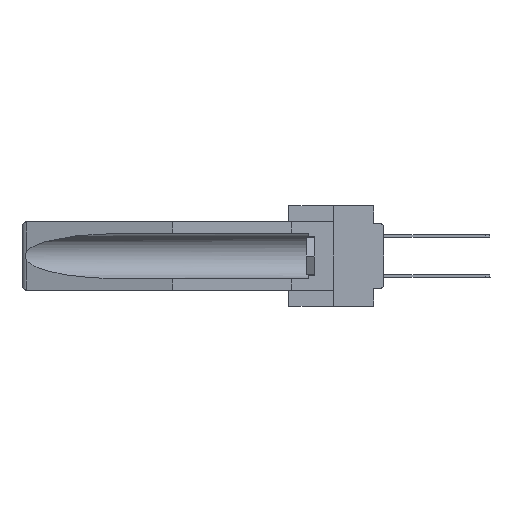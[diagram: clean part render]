
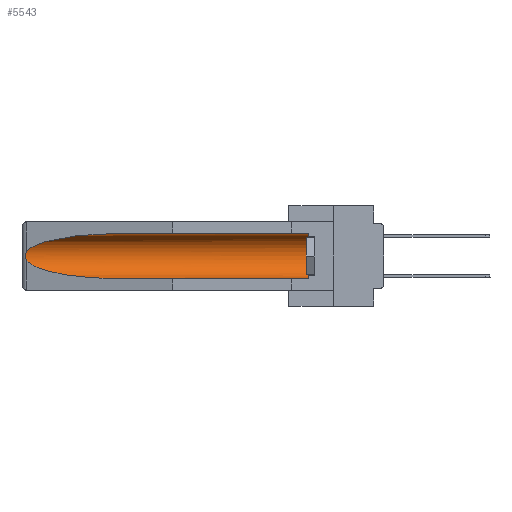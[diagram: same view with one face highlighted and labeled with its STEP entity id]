
A CAD part, left-side view. The second image highlights one B-rep face of the part: STEP entity #5543.
In plain terms, the highlighted cylindrical face has radius 2.857 mm (diameter 5.715 mm), a partial arc.
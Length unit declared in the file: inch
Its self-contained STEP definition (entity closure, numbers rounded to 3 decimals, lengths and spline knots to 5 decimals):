
#27 = DIRECTION ( 'NONE',  ( 0., 0., 1. ) ) ;
#2218 =( BOUNDED_CURVE ( )  B_SPLINE_CURVE ( 3, ( #14379, #23563, #2888, #16909 ),
 .UNSPECIFIED., .F., .F. ) 
 B_SPLINE_CURVE_WITH_KNOTS ( ( 4, 4 ),
 ( 4.71239, 6.08839 ),
 .UNSPECIFIED. ) 
 CURVE ( )  GEOMETRIC_REPRESENTATION_ITEM ( )  RATIONAL_B_SPLINE_CURVE ( ( 1., 0.848, 0.848, 1. ) ) 
 REPRESENTATION_ITEM ( '' )  );
#2528 = DIRECTION ( 'NONE',  ( 0., 1., 0. ) ) ;
#2888 = CARTESIAN_POINT ( 'NONE',  ( 0.25451, 1.48313, -0.09465 ) ) ;
#2907 = CARTESIAN_POINT ( 'NONE',  ( 0.155, 0.126, -0.284 ) ) ;
#2957 = CARTESIAN_POINT ( 'NONE',  ( 0.2673, 1.5327, -0.16383 ) ) ;
#3835 = CARTESIAN_POINT ( 'NONE',  ( 0.21114, 1.30732, -0.284 ) ) ;
#3884 = AXIS2_PLACEMENT_3D ( 'NONE', #9482, #20951, #7510 ) ;
#4705 = ORIENTED_EDGE ( 'NONE', *, *, #16435, .T. ) ;
#5543 = ADVANCED_FACE ( 'NONE', ( #10087 ), #23655, .F. ) ;
#5927 = ORIENTED_EDGE ( 'NONE', *, *, #19386, .T. ) ;
#6537 = CARTESIAN_POINT ( 'NONE',  ( 0.26537, 1.52718, -0.19328 ) ) ;
#7510 = DIRECTION ( 'NONE',  ( 0., 0., 1. ) ) ;
#8343 = VERTEX_POINT ( 'NONE', #20772 ) ;
#9447 = CARTESIAN_POINT ( 'NONE',  ( 0.2673, 1.53269, -0.17917 ) ) ;
#9482 = CARTESIAN_POINT ( 'NONE',  ( 0.155, -0.30754, -0.1715 ) ) ;
#10087 = FACE_OUTER_BOUND ( 'NONE', #13048, .T. ) ;
#10198 = CARTESIAN_POINT ( 'NONE',  ( 0.155, 1.07973, -0.284 ) ) ;
#10650 = CARTESIAN_POINT ( 'NONE',  ( 0.25451, 1.48313, -0.24835 ) ) ;
#11109 = ORIENTED_EDGE ( 'NONE', *, *, #19622, .T. ) ;
#11564 = CARTESIAN_POINT ( 'NONE',  ( 0.26537, 1.52718, -0.14972 ) ) ;
#11588 = CARTESIAN_POINT ( 'NONE',  ( 0.155, -0.30754, -0.284 ) ) ;
#11968 = CARTESIAN_POINT ( 'NONE',  ( 0.155, 1.07973, -0.059 ) ) ;
#12041 = VERTEX_POINT ( 'NONE', #11968 ) ;
#12634 = EDGE_CURVE ( 'NONE', #12041, #8343, #2218, .T. ) ;
#13048 = EDGE_LOOP ( 'NONE', ( #24551, #5927, #20894, #14125, #4705, #11109 ) ) ;
#13077 = CARTESIAN_POINT ( 'NONE',  ( 0.155, -0.30754, -0.059 ) ) ;
#14125 = ORIENTED_EDGE ( 'NONE', *, *, #14390, .F. ) ;
#14150 = CARTESIAN_POINT ( 'NONE',  ( 0.2675, 1.53308, -0.16763 ) ) ;
#14310 = VERTEX_POINT ( 'NONE', #20199 ) ;
#14379 = CARTESIAN_POINT ( 'NONE',  ( 0.155, 1.07973, -0.059 ) ) ;
#14390 = EDGE_CURVE ( 'NONE', #26250, #16099, #29537, .T. ) ;
#14656 = VECTOR ( 'NONE', #24506, 39.37008 ) ;
#14728 = CARTESIAN_POINT ( 'NONE',  ( 0.26537, 1.52718, -0.19328 ) ) ;
#16099 = VERTEX_POINT ( 'NONE', #20317 ) ;
#16199 = AXIS2_PLACEMENT_3D ( 'NONE', #29336, #27376, #27 ) ;
#16435 = EDGE_CURVE ( 'NONE', #26250, #14310, #16673, .T. ) ;
#16673 = CIRCLE ( 'NONE', #16199, 0.1125 ) ;
#16679 = CARTESIAN_POINT ( 'NONE',  ( 0.26597, 1.52961, -0.15275 ) ) ;
#16909 = CARTESIAN_POINT ( 'NONE',  ( 0.26537, 1.52718, -0.14972 ) ) ;
#17806 = B_SPLINE_CURVE_WITH_KNOTS ( 'NONE', 3,
 ( #11564, #16679, #23625, #2957, #14150, #25286, #9447, #20624, #29815, #18813 ),
 .UNSPECIFIED., .F., .F.,
 ( 4, 2, 2, 2, 4 ),
 ( 0., 0.00029, 0.00058, 0.00087, 0.00117 ),
 .UNSPECIFIED. ) ;
#18813 = CARTESIAN_POINT ( 'NONE',  ( 0.26537, 1.52718, -0.19328 ) ) ;
#19386 = EDGE_CURVE ( 'NONE', #8343, #27546, #17806, .T. ) ;
#19622 = EDGE_CURVE ( 'NONE', #14310, #12041, #20143, .T. ) ;
#20143 = LINE ( 'NONE', #13077, #14656 ) ;
#20199 = CARTESIAN_POINT ( 'NONE',  ( 0.155, 0.126, -0.059 ) ) ;
#20317 = CARTESIAN_POINT ( 'NONE',  ( 0.155, 1.07973, -0.284 ) ) ;
#20624 = CARTESIAN_POINT ( 'NONE',  ( 0.26655, 1.53094, -0.18657 ) ) ;
#20772 = CARTESIAN_POINT ( 'NONE',  ( 0.26537, 1.52718, -0.14972 ) ) ;
#20894 = ORIENTED_EDGE ( 'NONE', *, *, #28941, .T. ) ;
#20951 = DIRECTION ( 'NONE',  ( 0., 1., 0. ) ) ;
#23563 = CARTESIAN_POINT ( 'NONE',  ( 0.21114, 1.30732, -0.059 ) ) ;
#23625 = CARTESIAN_POINT ( 'NONE',  ( 0.26654, 1.53092, -0.15636 ) ) ;
#23655 = CYLINDRICAL_SURFACE ( 'NONE', #3884, 0.1125 ) ;
#24001 =( BOUNDED_CURVE ( )  B_SPLINE_CURVE ( 3, ( #14728, #10650, #3835, #10198 ),
 .UNSPECIFIED., .F., .F. ) 
 B_SPLINE_CURVE_WITH_KNOTS ( ( 4, 4 ),
 ( 0.1948, 1.5708 ),
 .UNSPECIFIED. ) 
 CURVE ( )  GEOMETRIC_REPRESENTATION_ITEM ( )  RATIONAL_B_SPLINE_CURVE ( ( 1., 0.848, 0.848, 1. ) ) 
 REPRESENTATION_ITEM ( '' )  );
#24506 = DIRECTION ( 'NONE',  ( 0., 1., 0. ) ) ;
#24551 = ORIENTED_EDGE ( 'NONE', *, *, #12634, .T. ) ;
#25286 = CARTESIAN_POINT ( 'NONE',  ( 0.2675, 1.53308, -0.17534 ) ) ;
#25802 = VECTOR ( 'NONE', #2528, 39.37008 ) ;
#26250 = VERTEX_POINT ( 'NONE', #2907 ) ;
#27376 = DIRECTION ( 'NONE',  ( 0., -1., 0. ) ) ;
#27546 = VERTEX_POINT ( 'NONE', #6537 ) ;
#28941 = EDGE_CURVE ( 'NONE', #27546, #16099, #24001, .T. ) ;
#29336 = CARTESIAN_POINT ( 'NONE',  ( 0.155, 0.126, -0.1715 ) ) ;
#29537 = LINE ( 'NONE', #11588, #25802 ) ;
#29815 = CARTESIAN_POINT ( 'NONE',  ( 0.26597, 1.5296, -0.19026 ) ) ;
